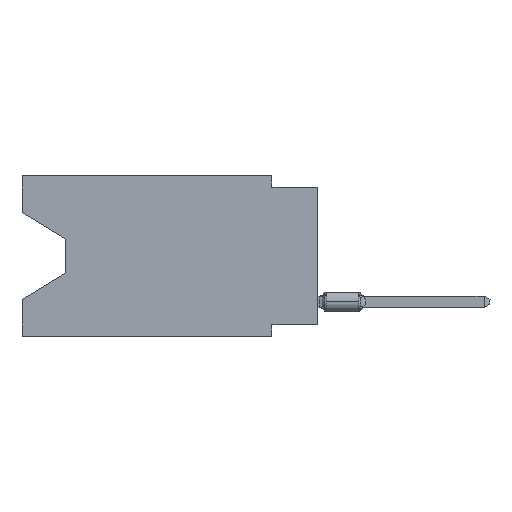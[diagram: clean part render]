
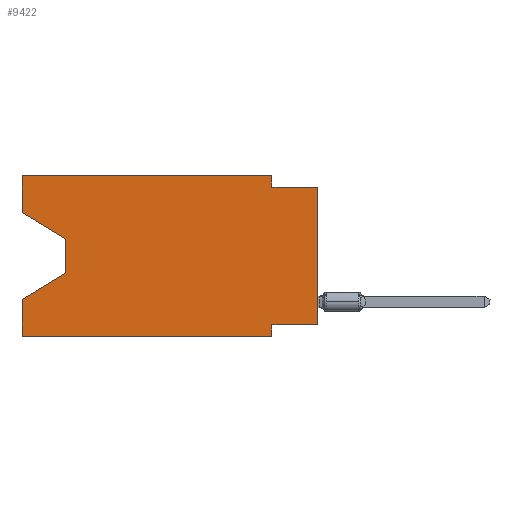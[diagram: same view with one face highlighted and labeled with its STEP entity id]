
A CAD part, left-side view. The second image highlights one B-rep face of the part: STEP entity #9422.
In plain terms, the highlighted planar face has unit normal (-1, 0, 0).
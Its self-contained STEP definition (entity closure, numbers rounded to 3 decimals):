
#128 = DIRECTION ( 'NONE',  ( 1., 0., 0. ) ) ;
#565 = ORIENTED_EDGE ( 'NONE', *, *, #27124, .F. ) ;
#810 = ORIENTED_EDGE ( 'NONE', *, *, #7265, .F. ) ;
#830 = CARTESIAN_POINT ( 'NONE',  ( 0., 13.97, -5.385 ) ) ;
#1498 = CARTESIAN_POINT ( 'NONE',  ( 0., 16.383, 0. ) ) ;
#2570 = VERTEX_POINT ( 'NONE', #21977 ) ;
#2592 = VERTEX_POINT ( 'NONE', #9716 ) ;
#2593 = VECTOR ( 'NONE', #28871, 1000. ) ;
#2851 = ORIENTED_EDGE ( 'NONE', *, *, #18520, .T. ) ;
#3320 = ORIENTED_EDGE ( 'NONE', *, *, #13166, .F. ) ;
#3634 = LINE ( 'NONE', #20355, #12941 ) ;
#3774 = EDGE_CURVE ( 'NONE', #23367, #23801, #8945, .T. ) ;
#4270 = VERTEX_POINT ( 'NONE', #6215 ) ;
#5387 = CARTESIAN_POINT ( 'NONE',  ( 0., 2.54, -8.89 ) ) ;
#5548 = CARTESIAN_POINT ( 'NONE',  ( 0., 16.383, -2.038 ) ) ;
#6215 = CARTESIAN_POINT ( 'NONE',  ( 0., 13.97, -5.385 ) ) ;
#6280 = LINE ( 'NONE', #1498, #20833 ) ;
#6929 = CARTESIAN_POINT ( 'NONE',  ( 0., 16.383, -2.038 ) ) ;
#7225 = EDGE_CURVE ( 'NONE', #16937, #2592, #17658, .T. ) ;
#7265 = EDGE_CURVE ( 'NONE', #28749, #8015, #27236, .T. ) ;
#7304 = EDGE_CURVE ( 'NONE', #2570, #16937, #30580, .T. ) ;
#8015 = VERTEX_POINT ( 'NONE', #28068 ) ;
#8404 = VECTOR ( 'NONE', #27084, 1000. ) ;
#8421 = CARTESIAN_POINT ( 'NONE',  ( 0., 2.54, 0. ) ) ;
#8945 = LINE ( 'NONE', #16428, #2593 ) ;
#9380 = CARTESIAN_POINT ( 'NONE',  ( 0., 13.97, -3.505 ) ) ;
#9422 = ADVANCED_FACE ( 'NONE', ( #12103 ), #26480, .F. ) ;
#9714 = VECTOR ( 'NONE', #21582, 1000. ) ;
#9716 = CARTESIAN_POINT ( 'NONE',  ( 0., 2.54, -0.635 ) ) ;
#9892 = CARTESIAN_POINT ( 'NONE',  ( 0., 0., -0.635 ) ) ;
#10047 = LINE ( 'NONE', #6929, #9714 ) ;
#10651 = LINE ( 'NONE', #15397, #30046 ) ;
#11053 = EDGE_CURVE ( 'NONE', #28475, #4270, #14167, .T. ) ;
#11229 = DIRECTION ( 'NONE',  ( 0., 0., 1. ) ) ;
#11881 = LINE ( 'NONE', #21764, #25874 ) ;
#12103 = FACE_OUTER_BOUND ( 'NONE', #27831, .T. ) ;
#12920 = VERTEX_POINT ( 'NONE', #5548 ) ;
#12941 = VECTOR ( 'NONE', #16039, 1000. ) ;
#13166 = EDGE_CURVE ( 'NONE', #12920, #2570, #6280, .T. ) ;
#13626 = ORIENTED_EDGE ( 'NONE', *, *, #3774, .T. ) ;
#13919 = ORIENTED_EDGE ( 'NONE', *, *, #19160, .F. ) ;
#13988 = DIRECTION ( 'NONE',  ( 0., -1., 0. ) ) ;
#14123 = CARTESIAN_POINT ( 'NONE',  ( 0., 2.54, -8.255 ) ) ;
#14167 = LINE ( 'NONE', #9380, #24793 ) ;
#14430 = ORIENTED_EDGE ( 'NONE', *, *, #17181, .T. ) ;
#15397 = CARTESIAN_POINT ( 'NONE',  ( 0., 0., -8.255 ) ) ;
#15569 = VERTEX_POINT ( 'NONE', #25680 ) ;
#16039 = DIRECTION ( 'NONE',  ( 0., -1., 0. ) ) ;
#16428 = CARTESIAN_POINT ( 'NONE',  ( 0., 0., 0. ) ) ;
#16937 = VERTEX_POINT ( 'NONE', #28592 ) ;
#17181 = EDGE_CURVE ( 'NONE', #15569, #8015, #24404, .T. ) ;
#17658 = LINE ( 'NONE', #8421, #8404 ) ;
#17897 = LINE ( 'NONE', #830, #25980 ) ;
#18456 = CARTESIAN_POINT ( 'NONE',  ( 0., 16.383, 0. ) ) ;
#18520 = EDGE_CURVE ( 'NONE', #4270, #29363, #17897, .T. ) ;
#18620 = VECTOR ( 'NONE', #13988, 1000. ) ;
#18771 = VECTOR ( 'NONE', #30136, 1000. ) ;
#19082 = DIRECTION ( 'NONE',  ( 0., 0., -1. ) ) ;
#19160 = EDGE_CURVE ( 'NONE', #23367, #28749, #10651, .T. ) ;
#19426 = DIRECTION ( 'NONE',  ( 0., 0., -1. ) ) ;
#19735 = EDGE_CURVE ( 'NONE', #12920, #28475, #10047, .T. ) ;
#19961 = DIRECTION ( 'NONE',  ( 0., 0.855, -0.519 ) ) ;
#20355 = CARTESIAN_POINT ( 'NONE',  ( 0., 0., -0.635 ) ) ;
#20833 = VECTOR ( 'NONE', #11229, 1000. ) ;
#21582 = DIRECTION ( 'NONE',  ( 0., -0.855, -0.519 ) ) ;
#21589 = CARTESIAN_POINT ( 'NONE',  ( 0., 0., -8.255 ) ) ;
#21669 = CARTESIAN_POINT ( 'NONE',  ( 0., 16.383, 0. ) ) ;
#21683 = AXIS2_PLACEMENT_3D ( 'NONE', #21669, #128, #19426 ) ;
#21764 = CARTESIAN_POINT ( 'NONE',  ( 0., 16.383, 0. ) ) ;
#21977 = CARTESIAN_POINT ( 'NONE',  ( 0., 16.383, 0. ) ) ;
#23093 = ORIENTED_EDGE ( 'NONE', *, *, #19735, .T. ) ;
#23367 = VERTEX_POINT ( 'NONE', #21589 ) ;
#23801 = VERTEX_POINT ( 'NONE', #9892 ) ;
#23863 = DIRECTION ( 'NONE',  ( 0., 0., 1. ) ) ;
#24404 = LINE ( 'NONE', #24880, #18771 ) ;
#24699 = VECTOR ( 'NONE', #27409, 1000. ) ;
#24793 = VECTOR ( 'NONE', #19082, 1000. ) ;
#24824 = DIRECTION ( 'NONE',  ( 0., 1., 0. ) ) ;
#24880 = CARTESIAN_POINT ( 'NONE',  ( 0., 16.383, -8.89 ) ) ;
#25285 = CARTESIAN_POINT ( 'NONE',  ( 0., 13.97, -3.505 ) ) ;
#25680 = CARTESIAN_POINT ( 'NONE',  ( 0., 16.383, -8.89 ) ) ;
#25874 = VECTOR ( 'NONE', #23863, 1000. ) ;
#25980 = VECTOR ( 'NONE', #19961, 1000. ) ;
#26065 = EDGE_CURVE ( 'NONE', #15569, #29363, #11881, .T. ) ;
#26480 = PLANE ( 'NONE',  #21683 ) ;
#27084 = DIRECTION ( 'NONE',  ( 0., 0., -1. ) ) ;
#27124 = EDGE_CURVE ( 'NONE', #2592, #23801, #3634, .T. ) ;
#27236 = LINE ( 'NONE', #5387, #24699 ) ;
#27409 = DIRECTION ( 'NONE',  ( 0., 0., -1. ) ) ;
#27831 = EDGE_LOOP ( 'NONE', ( #23093, #31281, #2851, #31157, #14430, #810, #13919, #13626, #565, #28981, #29018, #3320 ) ) ;
#28068 = CARTESIAN_POINT ( 'NONE',  ( 0., 2.54, -8.89 ) ) ;
#28475 = VERTEX_POINT ( 'NONE', #25285 ) ;
#28592 = CARTESIAN_POINT ( 'NONE',  ( 0., 2.54, 0. ) ) ;
#28749 = VERTEX_POINT ( 'NONE', #14123 ) ;
#28871 = DIRECTION ( 'NONE',  ( 0., 0., 1. ) ) ;
#28981 = ORIENTED_EDGE ( 'NONE', *, *, #7225, .F. ) ;
#29018 = ORIENTED_EDGE ( 'NONE', *, *, #7304, .F. ) ;
#29357 = CARTESIAN_POINT ( 'NONE',  ( 0., 16.383, -6.852 ) ) ;
#29363 = VERTEX_POINT ( 'NONE', #29357 ) ;
#30046 = VECTOR ( 'NONE', #24824, 1000. ) ;
#30136 = DIRECTION ( 'NONE',  ( 0., -1., 0. ) ) ;
#30580 = LINE ( 'NONE', #18456, #18620 ) ;
#31157 = ORIENTED_EDGE ( 'NONE', *, *, #26065, .F. ) ;
#31281 = ORIENTED_EDGE ( 'NONE', *, *, #11053, .T. ) ;
